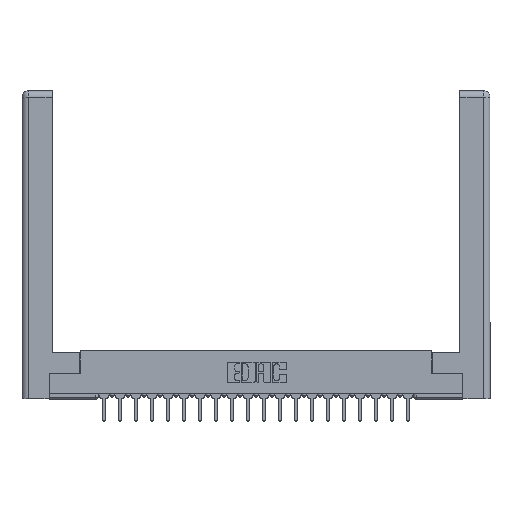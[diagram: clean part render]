
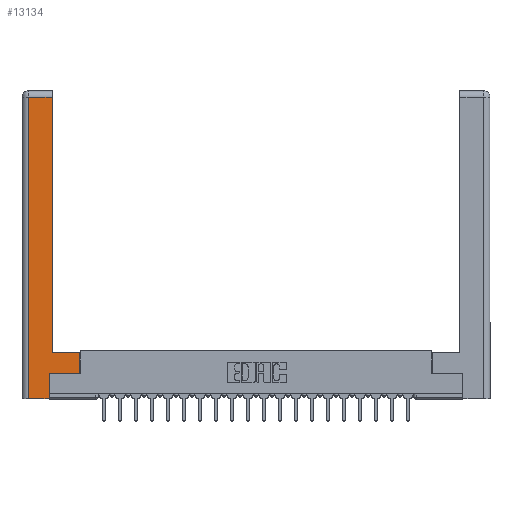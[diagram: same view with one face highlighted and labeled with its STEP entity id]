
A CAD part, top view. The second image highlights one B-rep face of the part: STEP entity #13134.
In plain terms, the highlighted planar face has unit normal (0, 0, 1).
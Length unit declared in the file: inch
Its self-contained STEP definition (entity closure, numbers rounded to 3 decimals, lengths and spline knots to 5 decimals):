
#186 = CARTESIAN_POINT ( 'NONE',  ( 0.565, 0.245, 0. ) ) ;
#670 = VECTOR ( 'NONE', #17841, 39.37008 ) ;
#915 = DIRECTION ( 'NONE',  ( 1., 0., 0. ) ) ;
#983 = DIRECTION ( 'NONE',  ( 0., 1., 0. ) ) ;
#1176 = VECTOR ( 'NONE', #15671, 39.37008 ) ;
#1767 = VECTOR ( 'NONE', #915, 39.37008 ) ;
#2034 = CARTESIAN_POINT ( 'NONE',  ( 0.265, 0.245, 0. ) ) ;
#2090 = ORIENTED_EDGE ( 'NONE', *, *, #7854, .T. ) ;
#2338 = VERTEX_POINT ( 'NONE', #17529 ) ;
#2412 = CARTESIAN_POINT ( 'NONE',  ( 0.0615, 0., 0. ) ) ;
#2482 = CARTESIAN_POINT ( 'NONE',  ( 0.295, 0.45, 0. ) ) ;
#2764 = CARTESIAN_POINT ( 'NONE',  ( 0.295, 2.94, 0. ) ) ;
#3179 = AXIS2_PLACEMENT_3D ( 'NONE', #9999, #21806, #21692 ) ;
#3733 = ORIENTED_EDGE ( 'NONE', *, *, #9881, .T. ) ;
#3875 = EDGE_CURVE ( 'NONE', #13718, #2338, #15017, .T. ) ;
#4130 = VECTOR ( 'NONE', #18797, 39.37008 ) ;
#4389 = CARTESIAN_POINT ( 'NONE',  ( 0.0615, 2.94, 0. ) ) ;
#4847 = ORIENTED_EDGE ( 'NONE', *, *, #7411, .T. ) ;
#4862 = CARTESIAN_POINT ( 'NONE',  ( 0.295, 0.45, 0. ) ) ;
#5148 = VECTOR ( 'NONE', #983, 39.37008 ) ;
#5574 = VERTEX_POINT ( 'NONE', #2482 ) ;
#5690 = ORIENTED_EDGE ( 'NONE', *, *, #3875, .T. ) ;
#6149 = ORIENTED_EDGE ( 'NONE', *, *, #13425, .T. ) ;
#6629 = EDGE_CURVE ( 'NONE', #17944, #5574, #8732, .T. ) ;
#6978 = ORIENTED_EDGE ( 'NONE', *, *, #6629, .T. ) ;
#7182 = CARTESIAN_POINT ( 'NONE',  ( 0.0615, 2.94, 0. ) ) ;
#7411 = EDGE_CURVE ( 'NONE', #18071, #20803, #10277, .T. ) ;
#7854 = EDGE_CURVE ( 'NONE', #9988, #13718, #15474, .T. ) ;
#7917 = CARTESIAN_POINT ( 'NONE',  ( 0.565, 0.45, 0. ) ) ;
#8197 = CARTESIAN_POINT ( 'NONE',  ( 0.0615, 0., 0. ) ) ;
#8212 = EDGE_CURVE ( 'NONE', #20803, #17944, #13364, .T. ) ;
#8732 = LINE ( 'NONE', #4862, #1176 ) ;
#9604 = DIRECTION ( 'NONE',  ( 0., 1., 0. ) ) ;
#9881 = EDGE_CURVE ( 'NONE', #5574, #20960, #18370, .T. ) ;
#9988 = VERTEX_POINT ( 'NONE', #4389 ) ;
#9999 = CARTESIAN_POINT ( 'NONE',  ( 0., 0., 0. ) ) ;
#10277 = LINE ( 'NONE', #13451, #4130 ) ;
#11023 = VECTOR ( 'NONE', #14848, 39.37008 ) ;
#11146 = CARTESIAN_POINT ( 'NONE',  ( 0.265, 0., 0. ) ) ;
#12884 = VECTOR ( 'NONE', #15127, 39.37008 ) ;
#13134 = ADVANCED_FACE ( 'NONE', ( #13408 ), #20220, .F. ) ;
#13364 = LINE ( 'NONE', #7917, #11023 ) ;
#13408 = FACE_OUTER_BOUND ( 'NONE', #19136, .T. ) ;
#13425 = EDGE_CURVE ( 'NONE', #2338, #18071, #19337, .T. ) ;
#13451 = CARTESIAN_POINT ( 'NONE',  ( 0.565, 0.245, 0. ) ) ;
#13718 = VERTEX_POINT ( 'NONE', #2412 ) ;
#14848 = DIRECTION ( 'NONE',  ( 0., 1., 0. ) ) ;
#14856 = CARTESIAN_POINT ( 'NONE',  ( 0.295, 3., 0. ) ) ;
#15017 = LINE ( 'NONE', #11146, #1767 ) ;
#15089 = EDGE_CURVE ( 'NONE', #20960, #9988, #21031, .T. ) ;
#15127 = DIRECTION ( 'NONE',  ( 0., -1., 0. ) ) ;
#15235 = ORIENTED_EDGE ( 'NONE', *, *, #15089, .T. ) ;
#15474 = LINE ( 'NONE', #8197, #12884 ) ;
#15671 = DIRECTION ( 'NONE',  ( -1., 0., 0. ) ) ;
#16638 = VECTOR ( 'NONE', #9604, 39.37008 ) ;
#17529 = CARTESIAN_POINT ( 'NONE',  ( 0.265, 0., 0. ) ) ;
#17561 = ORIENTED_EDGE ( 'NONE', *, *, #8212, .T. ) ;
#17841 = DIRECTION ( 'NONE',  ( -1., 0., 0. ) ) ;
#17944 = VERTEX_POINT ( 'NONE', #20124 ) ;
#18071 = VERTEX_POINT ( 'NONE', #21040 ) ;
#18370 = LINE ( 'NONE', #14856, #5148 ) ;
#18797 = DIRECTION ( 'NONE',  ( 1., 0., 0. ) ) ;
#19136 = EDGE_LOOP ( 'NONE', ( #3733, #15235, #2090, #5690, #6149, #4847, #17561, #6978 ) ) ;
#19337 = LINE ( 'NONE', #2034, #16638 ) ;
#20124 = CARTESIAN_POINT ( 'NONE',  ( 0.565, 0.45, 0. ) ) ;
#20220 = PLANE ( 'NONE',  #3179 ) ;
#20803 = VERTEX_POINT ( 'NONE', #186 ) ;
#20960 = VERTEX_POINT ( 'NONE', #2764 ) ;
#21031 = LINE ( 'NONE', #7182, #670 ) ;
#21040 = CARTESIAN_POINT ( 'NONE',  ( 0.265, 0.245, 0. ) ) ;
#21692 = DIRECTION ( 'NONE',  ( -1., 0., 0. ) ) ;
#21806 = DIRECTION ( 'NONE',  ( 0., 0., -1. ) ) ;
